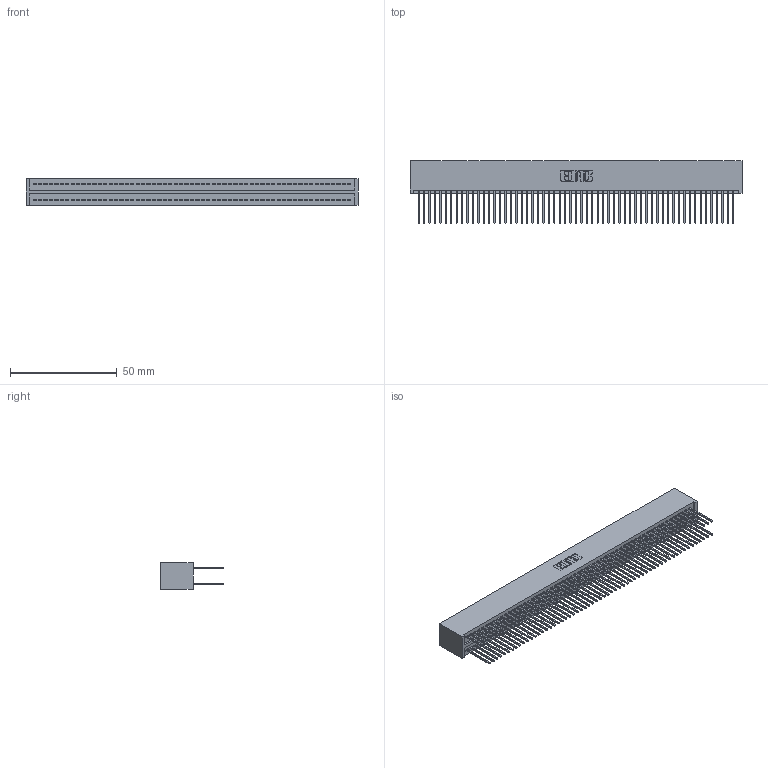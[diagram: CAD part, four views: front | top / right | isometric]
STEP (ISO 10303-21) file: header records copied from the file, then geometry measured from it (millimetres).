
FILE_DESCRIPTION (( 'STEP AP203' ), '1' );
FILE_NAME ('325-118-540-201.STEP', '2020-02-25T08:33:14', ( '' ), ( '' ), 'SwSTEP 2.0', 'SolidWorks 2016', '' );
FILE_SCHEMA (( 'CONFIG_CONTROL_DESIGN' ));
Length unit declared in the file: inch
Products named in the file (3): 325-292-001_325-293-140; 325-118-540-201; 325 Part_Lugless
Assembly tree (119 placements, depth 2):
  325-118-540-201
    325 Part_Lugless
    325-292-001_325-293-140  x118
Bounding box: 155.5 x 29.46 x 12.45 mm (x, y, z)
Volume: 21280.5 mm3; surface area: 28950.8 mm2
Topology: 119 solids, 119 shells, 6242 faces, 18577 edges, 12226 vertices
Faces by surface type: plane 4314, cylinder 1928
Entity records: 35499 total; most frequent: CARTESIAN_POINT 5862, ORIENTED_EDGE 5798, DIRECTION 4971, EDGE_CURVE 2899, LINE 2779, VECTOR 2779, VERTEX_POINT 1930, AXIS2_PLACEMENT_3D 1096
